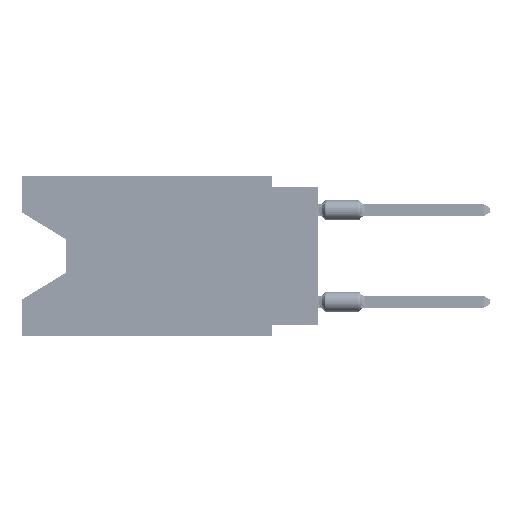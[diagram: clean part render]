
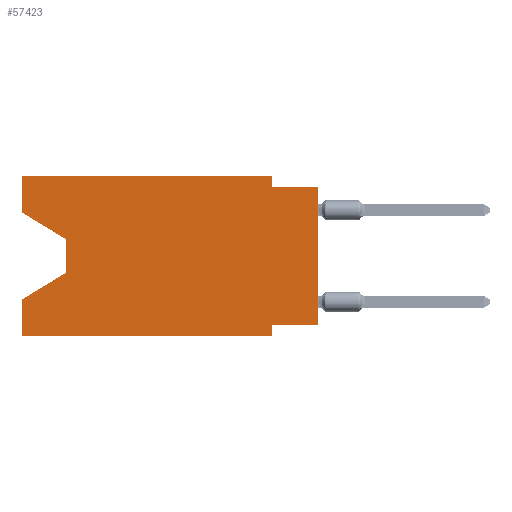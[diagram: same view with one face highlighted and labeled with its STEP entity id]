
A CAD part, left-side view. The second image highlights one B-rep face of the part: STEP entity #57423.
In plain terms, the highlighted planar face has unit normal (-1, 0, 0).
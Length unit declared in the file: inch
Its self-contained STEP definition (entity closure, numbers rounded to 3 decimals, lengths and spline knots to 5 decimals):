
#897 = CARTESIAN_POINT ( 'NONE',  ( 0., 0.645, 0. ) ) ;
#2022 = VERTEX_POINT ( 'NONE', #31197 ) ;
#2399 = LINE ( 'NONE', #16596, #63307 ) ;
#2969 = ORIENTED_EDGE ( 'NONE', *, *, #24963, .T. ) ;
#6229 = ORIENTED_EDGE ( 'NONE', *, *, #35783, .F. ) ;
#6302 = VERTEX_POINT ( 'NONE', #7365 ) ;
#7172 = EDGE_CURVE ( 'NONE', #35321, #49147, #68442, .T. ) ;
#7365 = CARTESIAN_POINT ( 'NONE',  ( 0., 0.1, -0.025 ) ) ;
#7492 = VERTEX_POINT ( 'NONE', #34042 ) ;
#9039 = DIRECTION ( 'NONE',  ( 1., 0., 0. ) ) ;
#9961 = DIRECTION ( 'NONE',  ( 0., 0., -1. ) ) ;
#11287 = DIRECTION ( 'NONE',  ( 0., -1., 0. ) ) ;
#11289 = EDGE_CURVE ( 'NONE', #15512, #7492, #49805, .T. ) ;
#11997 = ORIENTED_EDGE ( 'NONE', *, *, #41855, .F. ) ;
#15512 = VERTEX_POINT ( 'NONE', #36198 ) ;
#15694 = PLANE ( 'NONE',  #22640 ) ;
#16596 = CARTESIAN_POINT ( 'NONE',  ( 0., 0.645, -0.35 ) ) ;
#17078 = LINE ( 'NONE', #57496, #74660 ) ;
#17660 = CARTESIAN_POINT ( 'NONE',  ( 0., 0.645, 0. ) ) ;
#17822 = CARTESIAN_POINT ( 'NONE',  ( 0., 0.645, 0. ) ) ;
#18796 = ORIENTED_EDGE ( 'NONE', *, *, #76723, .T. ) ;
#19566 = LINE ( 'NONE', #897, #27981 ) ;
#20475 = ORIENTED_EDGE ( 'NONE', *, *, #39974, .T. ) ;
#21689 = ORIENTED_EDGE ( 'NONE', *, *, #79544, .F. ) ;
#21960 = VERTEX_POINT ( 'NONE', #45038 ) ;
#22594 = CARTESIAN_POINT ( 'NONE',  ( 0., 0.55, -0.138 ) ) ;
#22640 = AXIS2_PLACEMENT_3D ( 'NONE', #27706, #9039, #68114 ) ;
#23239 = CARTESIAN_POINT ( 'NONE',  ( 0., 0., -0.325 ) ) ;
#24963 = EDGE_CURVE ( 'NONE', #68264, #75278, #27344, .T. ) ;
#27308 = VECTOR ( 'NONE', #29772, 39.37008 ) ;
#27344 = LINE ( 'NONE', #41554, #73832 ) ;
#27457 = VECTOR ( 'NONE', #9961, 39.37008 ) ;
#27706 = CARTESIAN_POINT ( 'NONE',  ( 0., 0.645, 0. ) ) ;
#27981 = VECTOR ( 'NONE', #48404, 39.37008 ) ;
#29652 = ORIENTED_EDGE ( 'NONE', *, *, #7172, .T. ) ;
#29772 = DIRECTION ( 'NONE',  ( 0., 1., 0. ) ) ;
#29819 = LINE ( 'NONE', #17822, #59315 ) ;
#31197 = CARTESIAN_POINT ( 'NONE',  ( 0., 0.1, 0. ) ) ;
#32655 = ORIENTED_EDGE ( 'NONE', *, *, #11289, .T. ) ;
#34042 = CARTESIAN_POINT ( 'NONE',  ( 0., 0.645, -0.26975 ) ) ;
#35321 = VERTEX_POINT ( 'NONE', #23239 ) ;
#35692 = FACE_OUTER_BOUND ( 'NONE', #71108, .T. ) ;
#35783 = EDGE_CURVE ( 'NONE', #35321, #85669, #56448, .T. ) ;
#36198 = CARTESIAN_POINT ( 'NONE',  ( 0., 0.55, -0.212 ) ) ;
#36319 = CARTESIAN_POINT ( 'NONE',  ( 0., 0.1, -0.325 ) ) ;
#36803 = VECTOR ( 'NONE', #75536, 39.37008 ) ;
#38045 = CARTESIAN_POINT ( 'NONE',  ( 0., 0.645, -0.35 ) ) ;
#39974 = EDGE_CURVE ( 'NONE', #68646, #48145, #2399, .T. ) ;
#41554 = CARTESIAN_POINT ( 'NONE',  ( 0., 0.645, -0.08025 ) ) ;
#41855 = EDGE_CURVE ( 'NONE', #21960, #2022, #19566, .T. ) ;
#41964 = CARTESIAN_POINT ( 'NONE',  ( 0., 0.1, 0. ) ) ;
#42201 = ORIENTED_EDGE ( 'NONE', *, *, #69018, .F. ) ;
#44022 = DIRECTION ( 'NONE',  ( 0., 0.855, -0.519 ) ) ;
#45038 = CARTESIAN_POINT ( 'NONE',  ( 0., 0.645, 0. ) ) ;
#48145 = VERTEX_POINT ( 'NONE', #67477 ) ;
#48404 = DIRECTION ( 'NONE',  ( 0., -1., 0. ) ) ;
#49053 = LINE ( 'NONE', #41964, #27457 ) ;
#49147 = VERTEX_POINT ( 'NONE', #57345 ) ;
#49805 = LINE ( 'NONE', #76890, #84999 ) ;
#50185 = CARTESIAN_POINT ( 'NONE',  ( 0., 0.1, -0.35 ) ) ;
#52018 = DIRECTION ( 'NONE',  ( 0., 0., 1. ) ) ;
#53572 = DIRECTION ( 'NONE',  ( 0., -0.855, -0.519 ) ) ;
#54460 = ORIENTED_EDGE ( 'NONE', *, *, #82639, .F. ) ;
#55259 = ORIENTED_EDGE ( 'NONE', *, *, #82518, .F. ) ;
#56448 = LINE ( 'NONE', #82194, #27308 ) ;
#57345 = CARTESIAN_POINT ( 'NONE',  ( 0., 0., -0.025 ) ) ;
#57423 = ADVANCED_FACE ( 'NONE', ( #35692 ), #15694, .F. ) ;
#57496 = CARTESIAN_POINT ( 'NONE',  ( 0., 0., -0.025 ) ) ;
#58070 = LINE ( 'NONE', #17660, #67867 ) ;
#58681 = CARTESIAN_POINT ( 'NONE',  ( 0., 0.55, -0.138 ) ) ;
#59315 = VECTOR ( 'NONE', #52018, 39.37008 ) ;
#62216 = CARTESIAN_POINT ( 'NONE',  ( 0., 0., 0. ) ) ;
#63307 = VECTOR ( 'NONE', #70318, 39.37008 ) ;
#63729 = EDGE_CURVE ( 'NONE', #2022, #6302, #49053, .T. ) ;
#64723 = DIRECTION ( 'NONE',  ( 0., 0., 1. ) ) ;
#66869 = ORIENTED_EDGE ( 'NONE', *, *, #63729, .F. ) ;
#67477 = CARTESIAN_POINT ( 'NONE',  ( 0., 0.1, -0.35 ) ) ;
#67867 = VECTOR ( 'NONE', #64723, 39.37008 ) ;
#68114 = DIRECTION ( 'NONE',  ( 0., 0., -1. ) ) ;
#68264 = VERTEX_POINT ( 'NONE', #87070 ) ;
#68442 = LINE ( 'NONE', #62216, #36803 ) ;
#68646 = VERTEX_POINT ( 'NONE', #38045 ) ;
#69018 = EDGE_CURVE ( 'NONE', #6302, #49147, #17078, .T. ) ;
#70318 = DIRECTION ( 'NONE',  ( 0., -1., 0. ) ) ;
#71108 = EDGE_LOOP ( 'NONE', ( #2969, #18796, #32655, #55259, #20475, #21689, #6229, #29652, #42201, #66869, #11997, #54460 ) ) ;
#71554 = LINE ( 'NONE', #58681, #74474 ) ;
#73832 = VECTOR ( 'NONE', #53572, 39.37008 ) ;
#74474 = VECTOR ( 'NONE', #85750, 39.37008 ) ;
#74660 = VECTOR ( 'NONE', #11287, 39.37008 ) ;
#75278 = VERTEX_POINT ( 'NONE', #22594 ) ;
#75536 = DIRECTION ( 'NONE',  ( 0., 0., 1. ) ) ;
#75930 = LINE ( 'NONE', #50185, #84479 ) ;
#76723 = EDGE_CURVE ( 'NONE', #75278, #15512, #71554, .T. ) ;
#76890 = CARTESIAN_POINT ( 'NONE',  ( 0., 0.55, -0.212 ) ) ;
#79544 = EDGE_CURVE ( 'NONE', #85669, #48145, #75930, .T. ) ;
#82194 = CARTESIAN_POINT ( 'NONE',  ( 0., 0., -0.325 ) ) ;
#82518 = EDGE_CURVE ( 'NONE', #68646, #7492, #58070, .T. ) ;
#82639 = EDGE_CURVE ( 'NONE', #68264, #21960, #29819, .T. ) ;
#83025 = DIRECTION ( 'NONE',  ( 0., 0., -1. ) ) ;
#84479 = VECTOR ( 'NONE', #83025, 39.37008 ) ;
#84999 = VECTOR ( 'NONE', #44022, 39.37008 ) ;
#85669 = VERTEX_POINT ( 'NONE', #36319 ) ;
#85750 = DIRECTION ( 'NONE',  ( 0., 0., -1. ) ) ;
#87070 = CARTESIAN_POINT ( 'NONE',  ( 0., 0.645, -0.08025 ) ) ;
